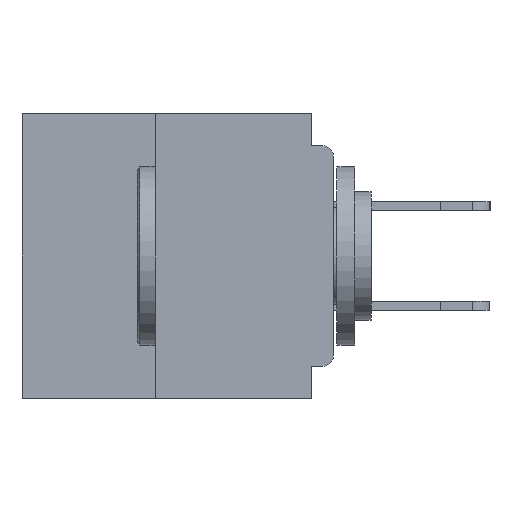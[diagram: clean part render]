
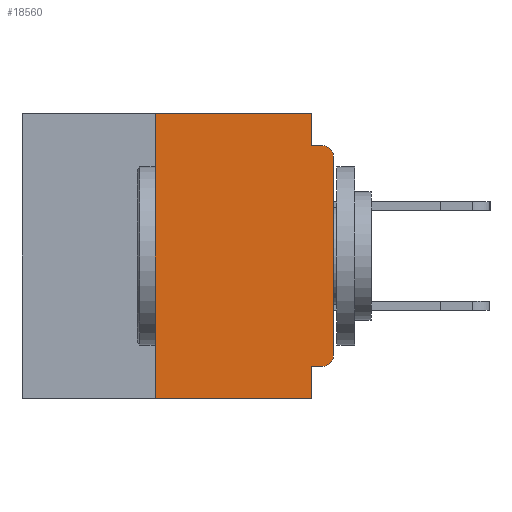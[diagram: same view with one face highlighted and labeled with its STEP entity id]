
A CAD part, left-side view. The second image highlights one B-rep face of the part: STEP entity #18560.
In plain terms, the highlighted planar face has unit normal (-1, 0, 0).
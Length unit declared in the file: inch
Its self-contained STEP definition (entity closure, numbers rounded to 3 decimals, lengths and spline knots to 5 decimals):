
#396 = CARTESIAN_POINT ( 'NONE',  ( 0., 0.25, 0. ) ) ;
#3120 = AXIS2_PLACEMENT_3D ( 'NONE', #19596, #52219, #24305 ) ;
#3694 = EDGE_CURVE ( 'NONE', #3737, #12145, #23770, .T. ) ;
#3737 = VERTEX_POINT ( 'NONE', #44230 ) ;
#4604 = EDGE_CURVE ( 'NONE', #26173, #41922, #38293, .T. ) ;
#4697 = CARTESIAN_POINT ( 'NONE',  ( 0., 0.437, -0.4 ) ) ;
#5322 = LINE ( 'NONE', #4697, #42607 ) ;
#6360 = LINE ( 'NONE', #47158, #31259 ) ;
#7354 = CARTESIAN_POINT ( 'NONE',  ( 0., 0., -0.355 ) ) ;
#7387 = CARTESIAN_POINT ( 'NONE',  ( 0., 0., -0.34 ) ) ;
#8838 = CARTESIAN_POINT ( 'NONE',  ( 0., 0.031, 0. ) ) ;
#8841 = EDGE_CURVE ( 'NONE', #52459, #17012, #20883, .T. ) ;
#9765 = LINE ( 'NONE', #17064, #20797 ) ;
#10282 = CARTESIAN_POINT ( 'NONE',  ( 0., 0.25, -0.4 ) ) ;
#10764 = ORIENTED_EDGE ( 'NONE', *, *, #33897, .T. ) ;
#12089 = DIRECTION ( 'NONE',  ( 0., 1., 0. ) ) ;
#12145 = VERTEX_POINT ( 'NONE', #7387 ) ;
#12317 = DIRECTION ( 'NONE',  ( 0., 0., -1. ) ) ;
#13067 = DIRECTION ( 'NONE',  ( 0., -1., 0. ) ) ;
#14718 = VECTOR ( 'NONE', #46222, 39.37008 ) ;
#15094 = CARTESIAN_POINT ( 'NONE',  ( 0., 0., -0.045 ) ) ;
#15550 = ORIENTED_EDGE ( 'NONE', *, *, #31835, .F. ) ;
#15691 = ORIENTED_EDGE ( 'NONE', *, *, #59903, .F. ) ;
#17012 = VERTEX_POINT ( 'NONE', #55468 ) ;
#17064 = CARTESIAN_POINT ( 'NONE',  ( 0., 0.25, -0.4 ) ) ;
#18560 = ADVANCED_FACE ( 'NONE', ( #58059 ), #35549, .F. ) ;
#19479 = AXIS2_PLACEMENT_3D ( 'NONE', #26239, #40256, #12317 ) ;
#19592 = ORIENTED_EDGE ( 'NONE', *, *, #22572, .T. ) ;
#19596 = CARTESIAN_POINT ( 'NONE',  ( 0., 0.015, -0.06 ) ) ;
#19828 = DIRECTION ( 'NONE',  ( 0., -1., 0. ) ) ;
#19989 = ORIENTED_EDGE ( 'NONE', *, *, #38040, .F. ) ;
#20176 = ORIENTED_EDGE ( 'NONE', *, *, #4604, .F. ) ;
#20724 = AXIS2_PLACEMENT_3D ( 'NONE', #53183, #25274, #57830 ) ;
#20797 = VECTOR ( 'NONE', #41143, 39.37008 ) ;
#20883 = LINE ( 'NONE', #15094, #44235 ) ;
#21570 = VECTOR ( 'NONE', #13067, 39.37008 ) ;
#22572 = EDGE_CURVE ( 'NONE', #42623, #17012, #48944, .T. ) ;
#23770 = CIRCLE ( 'NONE', #20724, 0.015 ) ;
#24013 = VECTOR ( 'NONE', #12089, 39.37008 ) ;
#24267 = LINE ( 'NONE', #8838, #14718 ) ;
#24305 = DIRECTION ( 'NONE',  ( 0., 0., -1. ) ) ;
#25274 = DIRECTION ( 'NONE',  ( -1., 0., 0. ) ) ;
#26173 = VERTEX_POINT ( 'NONE', #396 ) ;
#26239 = CARTESIAN_POINT ( 'NONE',  ( 0., 0.437, 0. ) ) ;
#31259 = VECTOR ( 'NONE', #51806, 39.37008 ) ;
#31659 = VERTEX_POINT ( 'NONE', #59532 ) ;
#31675 = CARTESIAN_POINT ( 'NONE',  ( 0., 0.437, 0. ) ) ;
#31835 = EDGE_CURVE ( 'NONE', #31659, #37280, #6360, .T. ) ;
#33565 = ORIENTED_EDGE ( 'NONE', *, *, #34937, .T. ) ;
#33897 = EDGE_CURVE ( 'NONE', #12145, #42623, #52967, .T. ) ;
#34937 = EDGE_CURVE ( 'NONE', #42386, #37280, #5322, .T. ) ;
#35049 = CARTESIAN_POINT ( 'NONE',  ( 0., 0.031, 0. ) ) ;
#35549 = PLANE ( 'NONE',  #19479 ) ;
#36340 = ORIENTED_EDGE ( 'NONE', *, *, #8841, .F. ) ;
#36366 = LINE ( 'NONE', #7354, #24013 ) ;
#37280 = VERTEX_POINT ( 'NONE', #44516 ) ;
#37887 = DIRECTION ( 'NONE',  ( 0., 0., 1. ) ) ;
#38040 = EDGE_CURVE ( 'NONE', #42386, #26173, #9765, .T. ) ;
#38293 = LINE ( 'NONE', #31675, #21570 ) ;
#40256 = DIRECTION ( 'NONE',  ( 1., 0., 0. ) ) ;
#41143 = DIRECTION ( 'NONE',  ( 0., 0., 1. ) ) ;
#41313 = EDGE_CURVE ( 'NONE', #3737, #31659, #36366, .T. ) ;
#41922 = VERTEX_POINT ( 'NONE', #35049 ) ;
#42386 = VERTEX_POINT ( 'NONE', #10282 ) ;
#42607 = VECTOR ( 'NONE', #46609, 39.37008 ) ;
#42618 = CARTESIAN_POINT ( 'NONE',  ( 0., 0., 0. ) ) ;
#42623 = VERTEX_POINT ( 'NONE', #49491 ) ;
#44230 = CARTESIAN_POINT ( 'NONE',  ( 0., 0.015, -0.355 ) ) ;
#44235 = VECTOR ( 'NONE', #19828, 39.37008 ) ;
#44516 = CARTESIAN_POINT ( 'NONE',  ( 0., 0.031, -0.4 ) ) ;
#46222 = DIRECTION ( 'NONE',  ( 0., 0., -1. ) ) ;
#46609 = DIRECTION ( 'NONE',  ( 0., -1., 0. ) ) ;
#47158 = CARTESIAN_POINT ( 'NONE',  ( 0., 0.031, -0.4 ) ) ;
#48361 = CARTESIAN_POINT ( 'NONE',  ( 0., 0.031, -0.045 ) ) ;
#48944 = CIRCLE ( 'NONE', #3120, 0.015 ) ;
#49491 = CARTESIAN_POINT ( 'NONE',  ( 0., 0., -0.06 ) ) ;
#50060 = VECTOR ( 'NONE', #37887, 39.37008 ) ;
#51806 = DIRECTION ( 'NONE',  ( 0., 0., -1. ) ) ;
#52219 = DIRECTION ( 'NONE',  ( -1., 0., 0. ) ) ;
#52459 = VERTEX_POINT ( 'NONE', #48361 ) ;
#52967 = LINE ( 'NONE', #42618, #50060 ) ;
#53183 = CARTESIAN_POINT ( 'NONE',  ( 0., 0.015, -0.34 ) ) ;
#55468 = CARTESIAN_POINT ( 'NONE',  ( 0., 0.015, -0.045 ) ) ;
#56011 = ORIENTED_EDGE ( 'NONE', *, *, #41313, .F. ) ;
#56349 = EDGE_LOOP ( 'NONE', ( #10764, #19592, #36340, #15691, #20176, #19989, #33565, #15550, #56011, #59953 ) ) ;
#57830 = DIRECTION ( 'NONE',  ( 0., 0., -1. ) ) ;
#58059 = FACE_OUTER_BOUND ( 'NONE', #56349, .T. ) ;
#59532 = CARTESIAN_POINT ( 'NONE',  ( 0., 0.031, -0.355 ) ) ;
#59903 = EDGE_CURVE ( 'NONE', #41922, #52459, #24267, .T. ) ;
#59953 = ORIENTED_EDGE ( 'NONE', *, *, #3694, .T. ) ;
